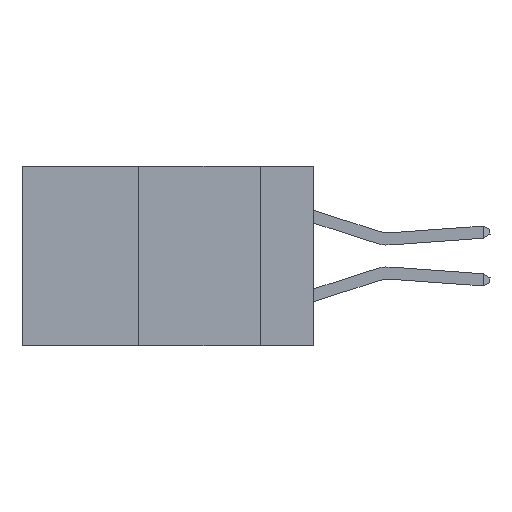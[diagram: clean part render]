
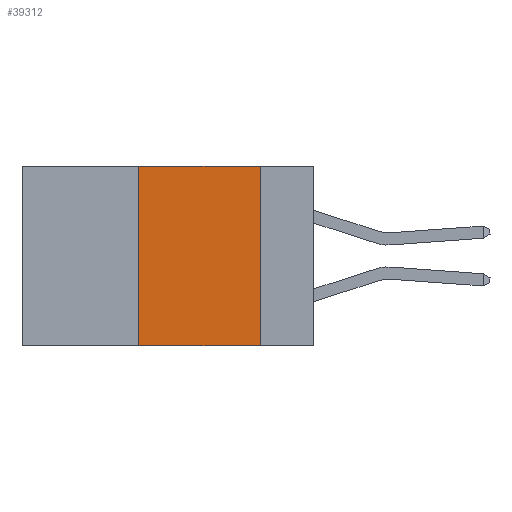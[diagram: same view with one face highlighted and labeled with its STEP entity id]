
A CAD part, left-side view. The second image highlights one B-rep face of the part: STEP entity #39312.
In plain terms, the highlighted planar face has unit normal (-1, 0, 0).
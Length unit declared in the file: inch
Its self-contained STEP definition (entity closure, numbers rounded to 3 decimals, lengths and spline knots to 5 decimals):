
#406 = LINE ( 'NONE', #4598, #16972 ) ;
#1331 = FACE_OUTER_BOUND ( 'NONE', #20399, .T. ) ;
#3604 = DIRECTION ( 'NONE',  ( 0., 0., 1. ) ) ;
#4577 = EDGE_CURVE ( 'NONE', #40802, #35820, #36986, .T. ) ;
#4598 = CARTESIAN_POINT ( 'NONE',  ( 0., 0.11, 0. ) ) ;
#4833 = DIRECTION ( 'NONE',  ( 1., 0., 0. ) ) ;
#6232 = VERTEX_POINT ( 'NONE', #22585 ) ;
#6554 = ORIENTED_EDGE ( 'NONE', *, *, #17279, .F. ) ;
#7429 = CARTESIAN_POINT ( 'NONE',  ( 0., 0.36, 0. ) ) ;
#7932 = CARTESIAN_POINT ( 'NONE',  ( 0., 0.11, -0.37 ) ) ;
#8605 = DIRECTION ( 'NONE',  ( 0., 0., -1. ) ) ;
#10050 = DIRECTION ( 'NONE',  ( 0., -1., 0. ) ) ;
#11525 = AXIS2_PLACEMENT_3D ( 'NONE', #22430, #4833, #8605 ) ;
#13645 = ORIENTED_EDGE ( 'NONE', *, *, #31080, .F. ) ;
#14570 = VERTEX_POINT ( 'NONE', #32899 ) ;
#16972 = VECTOR ( 'NONE', #42751, 39.37008 ) ;
#17279 = EDGE_CURVE ( 'NONE', #14570, #35820, #406, .T. ) ;
#17342 = EDGE_CURVE ( 'NONE', #6232, #14570, #43333, .T. ) ;
#18274 = LINE ( 'NONE', #7429, #31480 ) ;
#20399 = EDGE_LOOP ( 'NONE', ( #6554, #29581, #13645, #24638 ) ) ;
#20805 = CARTESIAN_POINT ( 'NONE',  ( 0., 0.36, -0.37 ) ) ;
#22037 = CARTESIAN_POINT ( 'NONE',  ( 0., 0.6, 0. ) ) ;
#22430 = CARTESIAN_POINT ( 'NONE',  ( 0., 0.6, 0. ) ) ;
#22585 = CARTESIAN_POINT ( 'NONE',  ( 0., 0.36, 0. ) ) ;
#24638 = ORIENTED_EDGE ( 'NONE', *, *, #4577, .T. ) ;
#27677 = CARTESIAN_POINT ( 'NONE',  ( 0., 0.6, -0.37 ) ) ;
#29030 = PLANE ( 'NONE',  #11525 ) ;
#29581 = ORIENTED_EDGE ( 'NONE', *, *, #17342, .F. ) ;
#31080 = EDGE_CURVE ( 'NONE', #40802, #6232, #18274, .T. ) ;
#31480 = VECTOR ( 'NONE', #3604, 39.37008 ) ;
#32899 = CARTESIAN_POINT ( 'NONE',  ( 0., 0.11, 0. ) ) ;
#34009 = VECTOR ( 'NONE', #43216, 39.37008 ) ;
#35820 = VERTEX_POINT ( 'NONE', #7932 ) ;
#35887 = VECTOR ( 'NONE', #10050, 39.37008 ) ;
#36986 = LINE ( 'NONE', #27677, #35887 ) ;
#39312 = ADVANCED_FACE ( 'NONE', ( #1331 ), #29030, .F. ) ;
#40802 = VERTEX_POINT ( 'NONE', #20805 ) ;
#42751 = DIRECTION ( 'NONE',  ( 0., 0., -1. ) ) ;
#43216 = DIRECTION ( 'NONE',  ( 0., -1., 0. ) ) ;
#43333 = LINE ( 'NONE', #22037, #34009 ) ;
